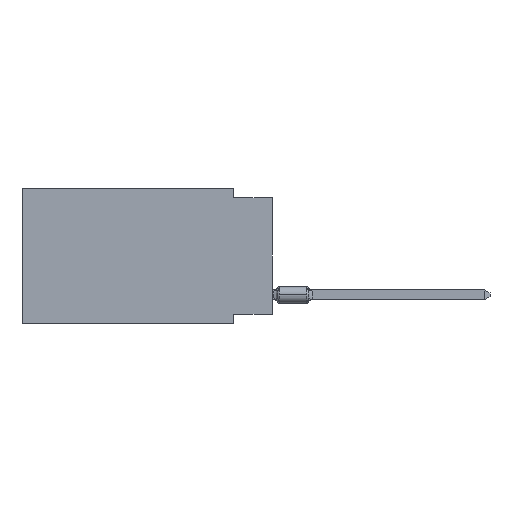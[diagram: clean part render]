
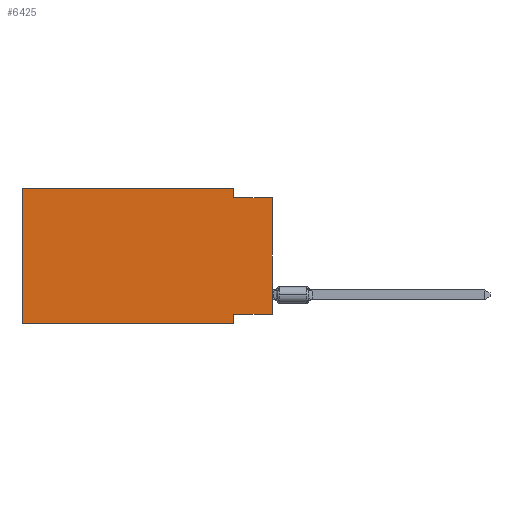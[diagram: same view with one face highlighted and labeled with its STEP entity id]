
A CAD part, left-side view. The second image highlights one B-rep face of the part: STEP entity #6425.
In plain terms, the highlighted planar face has unit normal (-1, 0, 0).
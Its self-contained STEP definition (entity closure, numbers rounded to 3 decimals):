
#116 = VECTOR ( 'NONE', #6601, 1000. ) ;
#136 = ORIENTED_EDGE ( 'NONE', *, *, #8543, .F. ) ;
#479 = EDGE_CURVE ( 'NONE', #2012, #9140, #4967, .T. ) ;
#668 = LINE ( 'NONE', #5235, #6256 ) ;
#853 = DIRECTION ( 'NONE',  ( 1., 0., 0. ) ) ;
#898 = LINE ( 'NONE', #14876, #10646 ) ;
#928 = FACE_OUTER_BOUND ( 'NONE', #6870, .T. ) ;
#1599 = CARTESIAN_POINT ( 'NONE',  ( 0., 0., -0.635 ) ) ;
#1753 = EDGE_CURVE ( 'NONE', #2012, #14680, #3069, .T. ) ;
#2012 = VERTEX_POINT ( 'NONE', #8372 ) ;
#2286 = ORIENTED_EDGE ( 'NONE', *, *, #1753, .T. ) ;
#2408 = VECTOR ( 'NONE', #11851, 1000. ) ;
#2514 = CARTESIAN_POINT ( 'NONE',  ( 0., 0., -8.255 ) ) ;
#2589 = CARTESIAN_POINT ( 'NONE',  ( 0., 16.383, 0. ) ) ;
#2648 = EDGE_CURVE ( 'NONE', #11784, #8465, #3033, .T. ) ;
#2771 = VERTEX_POINT ( 'NONE', #5828 ) ;
#2935 = DIRECTION ( 'NONE',  ( 0., 0., -1. ) ) ;
#3033 = LINE ( 'NONE', #7732, #116 ) ;
#3069 = LINE ( 'NONE', #11406, #9909 ) ;
#3319 = LINE ( 'NONE', #9021, #8442 ) ;
#3980 = VERTEX_POINT ( 'NONE', #4072 ) ;
#4072 = CARTESIAN_POINT ( 'NONE',  ( 0., 2.54, -8.255 ) ) ;
#4287 = ORIENTED_EDGE ( 'NONE', *, *, #2648, .F. ) ;
#4627 = EDGE_CURVE ( 'NONE', #3980, #14680, #7032, .T. ) ;
#4762 = CARTESIAN_POINT ( 'NONE',  ( 0., 2.54, -0.635 ) ) ;
#4967 = LINE ( 'NONE', #9757, #11603 ) ;
#5023 = VECTOR ( 'NONE', #13933, 1000. ) ;
#5235 = CARTESIAN_POINT ( 'NONE',  ( 0., 0., -8.255 ) ) ;
#5284 = AXIS2_PLACEMENT_3D ( 'NONE', #6635, #853, #2935 ) ;
#5489 = EDGE_CURVE ( 'NONE', #12656, #3980, #668, .T. ) ;
#5674 = EDGE_CURVE ( 'NONE', #2771, #11784, #3319, .T. ) ;
#5828 = CARTESIAN_POINT ( 'NONE',  ( 0., 2.54, 0. ) ) ;
#6256 = VECTOR ( 'NONE', #13126, 1000. ) ;
#6425 = ADVANCED_FACE ( 'NONE', ( #928 ), #11191, .F. ) ;
#6601 = DIRECTION ( 'NONE',  ( 0., -1., 0. ) ) ;
#6635 = CARTESIAN_POINT ( 'NONE',  ( 0., 16.383, 0. ) ) ;
#6870 = EDGE_LOOP ( 'NONE', ( #7238, #4287, #7132, #136, #10882, #2286, #7487, #13524 ) ) ;
#7032 = LINE ( 'NONE', #12712, #5023 ) ;
#7132 = ORIENTED_EDGE ( 'NONE', *, *, #5674, .F. ) ;
#7238 = ORIENTED_EDGE ( 'NONE', *, *, #7837, .T. ) ;
#7487 = ORIENTED_EDGE ( 'NONE', *, *, #4627, .F. ) ;
#7732 = CARTESIAN_POINT ( 'NONE',  ( 0., 0., -0.635 ) ) ;
#7773 = DIRECTION ( 'NONE',  ( 0., -1., 0. ) ) ;
#7837 = EDGE_CURVE ( 'NONE', #12656, #8465, #898, .T. ) ;
#8372 = CARTESIAN_POINT ( 'NONE',  ( 0., 16.383, -8.89 ) ) ;
#8442 = VECTOR ( 'NONE', #11437, 1000. ) ;
#8465 = VERTEX_POINT ( 'NONE', #1599 ) ;
#8543 = EDGE_CURVE ( 'NONE', #9140, #2771, #9878, .T. ) ;
#9021 = CARTESIAN_POINT ( 'NONE',  ( 0., 2.54, 0. ) ) ;
#9140 = VERTEX_POINT ( 'NONE', #13922 ) ;
#9757 = CARTESIAN_POINT ( 'NONE',  ( 0., 16.383, 0. ) ) ;
#9878 = LINE ( 'NONE', #2589, #2408 ) ;
#9909 = VECTOR ( 'NONE', #7773, 1000. ) ;
#10646 = VECTOR ( 'NONE', #11449, 1000. ) ;
#10690 = CARTESIAN_POINT ( 'NONE',  ( 0., 2.54, -8.89 ) ) ;
#10882 = ORIENTED_EDGE ( 'NONE', *, *, #479, .F. ) ;
#11191 = PLANE ( 'NONE',  #5284 ) ;
#11406 = CARTESIAN_POINT ( 'NONE',  ( 0., 16.383, -8.89 ) ) ;
#11437 = DIRECTION ( 'NONE',  ( 0., 0., -1. ) ) ;
#11449 = DIRECTION ( 'NONE',  ( 0., 0., 1. ) ) ;
#11603 = VECTOR ( 'NONE', #13225, 1000. ) ;
#11784 = VERTEX_POINT ( 'NONE', #4762 ) ;
#11851 = DIRECTION ( 'NONE',  ( 0., -1., 0. ) ) ;
#12656 = VERTEX_POINT ( 'NONE', #2514 ) ;
#12712 = CARTESIAN_POINT ( 'NONE',  ( 0., 2.54, -8.89 ) ) ;
#13126 = DIRECTION ( 'NONE',  ( 0., 1., 0. ) ) ;
#13225 = DIRECTION ( 'NONE',  ( 0., 0., 1. ) ) ;
#13524 = ORIENTED_EDGE ( 'NONE', *, *, #5489, .F. ) ;
#13922 = CARTESIAN_POINT ( 'NONE',  ( 0., 16.383, 0. ) ) ;
#13933 = DIRECTION ( 'NONE',  ( 0., 0., -1. ) ) ;
#14680 = VERTEX_POINT ( 'NONE', #10690 ) ;
#14876 = CARTESIAN_POINT ( 'NONE',  ( 0., 0., 0. ) ) ;
